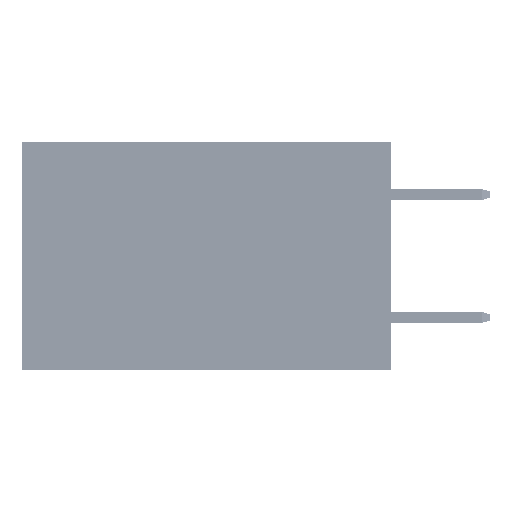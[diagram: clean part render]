
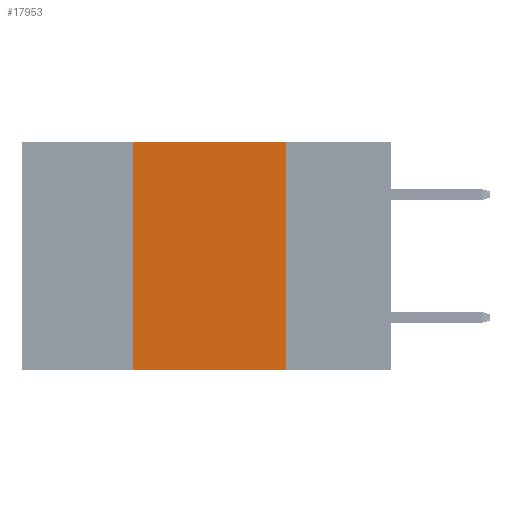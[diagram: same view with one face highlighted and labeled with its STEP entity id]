
A CAD part, left-side view. The second image highlights one B-rep face of the part: STEP entity #17953.
In plain terms, the highlighted planar face has unit normal (-1, 0, 0).
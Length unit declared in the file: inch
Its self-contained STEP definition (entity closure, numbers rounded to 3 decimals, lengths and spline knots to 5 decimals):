
#2117 = PLANE ( 'NONE',  #39336 ) ;
#2943 = ORIENTED_EDGE ( 'NONE', *, *, #26282, .F. ) ;
#7329 = CARTESIAN_POINT ( 'NONE',  ( 0., 0.17, 0. ) ) ;
#11294 = CARTESIAN_POINT ( 'NONE',  ( 0., 0.42, 0. ) ) ;
#13308 = DIRECTION ( 'NONE',  ( 0., -1., 0. ) ) ;
#13792 = CARTESIAN_POINT ( 'NONE',  ( 0., 0.6, 0. ) ) ;
#13951 = VECTOR ( 'NONE', #46365, 39.37008 ) ;
#14163 = VERTEX_POINT ( 'NONE', #32286 ) ;
#17281 = DIRECTION ( 'NONE',  ( 0., 0., -1. ) ) ;
#17486 = FACE_OUTER_BOUND ( 'NONE', #47728, .T. ) ;
#17521 = VECTOR ( 'NONE', #45453, 39.37008 ) ;
#17599 = EDGE_CURVE ( 'NONE', #27410, #30285, #38645, .T. ) ;
#17953 = ADVANCED_FACE ( 'NONE', ( #17486 ), #2117, .F. ) ;
#18526 = VERTEX_POINT ( 'NONE', #40885 ) ;
#19116 = DIRECTION ( 'NONE',  ( 0., 0., -1. ) ) ;
#19944 = LINE ( 'NONE', #21833, #17521 ) ;
#21833 = CARTESIAN_POINT ( 'NONE',  ( 0., 0.42, 0. ) ) ;
#23399 = CARTESIAN_POINT ( 'NONE',  ( 0., 0.6, 0. ) ) ;
#24119 = LINE ( 'NONE', #28771, #35572 ) ;
#24477 = ORIENTED_EDGE ( 'NONE', *, *, #17599, .F. ) ;
#25993 = EDGE_CURVE ( 'NONE', #14163, #18526, #24119, .T. ) ;
#26282 = EDGE_CURVE ( 'NONE', #30285, #18526, #30726, .T. ) ;
#27410 = VERTEX_POINT ( 'NONE', #11294 ) ;
#28771 = CARTESIAN_POINT ( 'NONE',  ( 0., 0.6, -0.37 ) ) ;
#30092 = EDGE_CURVE ( 'NONE', #14163, #27410, #19944, .T. ) ;
#30285 = VERTEX_POINT ( 'NONE', #7329 ) ;
#30726 = LINE ( 'NONE', #49849, #32516 ) ;
#32286 = CARTESIAN_POINT ( 'NONE',  ( 0., 0.42, -0.37 ) ) ;
#32516 = VECTOR ( 'NONE', #19116, 39.37008 ) ;
#35572 = VECTOR ( 'NONE', #13308, 39.37008 ) ;
#38645 = LINE ( 'NONE', #23399, #13951 ) ;
#39336 = AXIS2_PLACEMENT_3D ( 'NONE', #13792, #44650, #17281 ) ;
#40885 = CARTESIAN_POINT ( 'NONE',  ( 0., 0.17, -0.37 ) ) ;
#43540 = ORIENTED_EDGE ( 'NONE', *, *, #30092, .F. ) ;
#44650 = DIRECTION ( 'NONE',  ( 1., 0., 0. ) ) ;
#45453 = DIRECTION ( 'NONE',  ( 0., 0., 1. ) ) ;
#46365 = DIRECTION ( 'NONE',  ( 0., -1., 0. ) ) ;
#47728 = EDGE_LOOP ( 'NONE', ( #2943, #24477, #43540, #49456 ) ) ;
#49456 = ORIENTED_EDGE ( 'NONE', *, *, #25993, .T. ) ;
#49849 = CARTESIAN_POINT ( 'NONE',  ( 0., 0.17, 0. ) ) ;
